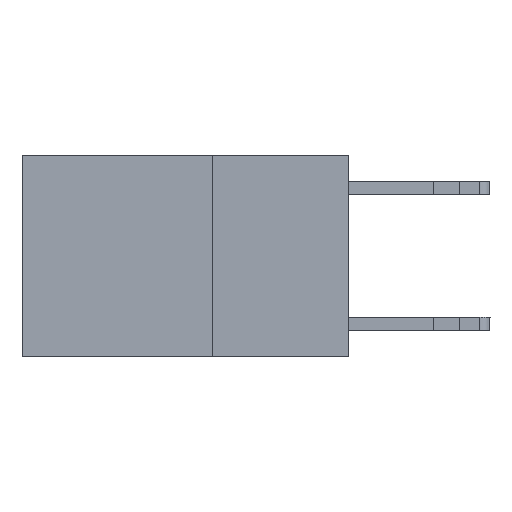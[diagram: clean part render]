
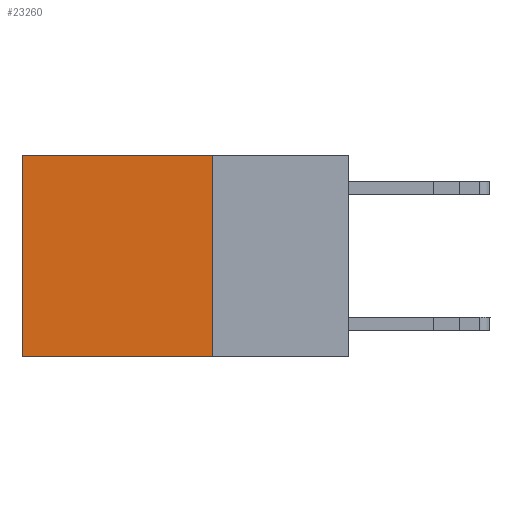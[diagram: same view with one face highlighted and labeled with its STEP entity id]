
A CAD part, left-side view. The second image highlights one B-rep face of the part: STEP entity #23260.
In plain terms, the highlighted planar face has unit normal (-1, 0, 0).
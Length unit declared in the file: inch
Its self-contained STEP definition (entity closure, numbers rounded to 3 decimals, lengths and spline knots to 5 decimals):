
#411 = DIRECTION ( 'NONE',  ( 0., 1., 0. ) ) ;
#1198 = CARTESIAN_POINT ( 'NONE',  ( 0.2625, 0.25, 0. ) ) ;
#1327 = VECTOR ( 'NONE', #5689, 39.37008 ) ;
#1967 = CARTESIAN_POINT ( 'NONE',  ( 0.2625, 0.6, 0. ) ) ;
#2812 = CARTESIAN_POINT ( 'NONE',  ( 0.2625, 0.25, 0. ) ) ;
#4085 = ORIENTED_EDGE ( 'NONE', *, *, #6502, .F. ) ;
#4603 = VECTOR ( 'NONE', #21632, 39.37008 ) ;
#5689 = DIRECTION ( 'NONE',  ( 0., 0., -1. ) ) ;
#6169 = CARTESIAN_POINT ( 'NONE',  ( 0.2625, 0.25, -0.37 ) ) ;
#6457 = CARTESIAN_POINT ( 'NONE',  ( 0.2625, 0.25, 0. ) ) ;
#6502 = EDGE_CURVE ( 'NONE', #11297, #17703, #17092, .T. ) ;
#7015 = ORIENTED_EDGE ( 'NONE', *, *, #15915, .T. ) ;
#9994 = VECTOR ( 'NONE', #411, 39.37008 ) ;
#11297 = VERTEX_POINT ( 'NONE', #6169 ) ;
#12090 = DIRECTION ( 'NONE',  ( 1., 0., 0. ) ) ;
#12906 = CARTESIAN_POINT ( 'NONE',  ( 0.2625, 0.6, -0.37 ) ) ;
#13787 = AXIS2_PLACEMENT_3D ( 'NONE', #19946, #12090, #26433 ) ;
#13802 = LINE ( 'NONE', #26238, #1327 ) ;
#14104 = PLANE ( 'NONE',  #13787 ) ;
#15061 = CARTESIAN_POINT ( 'NONE',  ( 0.2625, 0.25, -0.37 ) ) ;
#15638 = EDGE_LOOP ( 'NONE', ( #7015, #4085, #22061, #22293 ) ) ;
#15915 = EDGE_CURVE ( 'NONE', #21049, #17703, #13802, .T. ) ;
#17092 = LINE ( 'NONE', #15061, #9994 ) ;
#17703 = VERTEX_POINT ( 'NONE', #12906 ) ;
#18289 = VERTEX_POINT ( 'NONE', #1198 ) ;
#19946 = CARTESIAN_POINT ( 'NONE',  ( 0.2625, 0.25, 0. ) ) ;
#20077 = FACE_OUTER_BOUND ( 'NONE', #15638, .T. ) ;
#21023 = EDGE_CURVE ( 'NONE', #18289, #11297, #22412, .T. ) ;
#21049 = VERTEX_POINT ( 'NONE', #1967 ) ;
#21632 = DIRECTION ( 'NONE',  ( 0., 1., 0. ) ) ;
#22061 = ORIENTED_EDGE ( 'NONE', *, *, #21023, .F. ) ;
#22293 = ORIENTED_EDGE ( 'NONE', *, *, #23911, .T. ) ;
#22412 = LINE ( 'NONE', #6457, #25815 ) ;
#23260 = ADVANCED_FACE ( 'NONE', ( #20077 ), #14104, .F. ) ;
#23521 = LINE ( 'NONE', #2812, #4603 ) ;
#23911 = EDGE_CURVE ( 'NONE', #18289, #21049, #23521, .T. ) ;
#24839 = DIRECTION ( 'NONE',  ( 0., 0., -1. ) ) ;
#25815 = VECTOR ( 'NONE', #24839, 39.37008 ) ;
#26238 = CARTESIAN_POINT ( 'NONE',  ( 0.2625, 0.6, 0. ) ) ;
#26433 = DIRECTION ( 'NONE',  ( 0., 0., -1. ) ) ;
